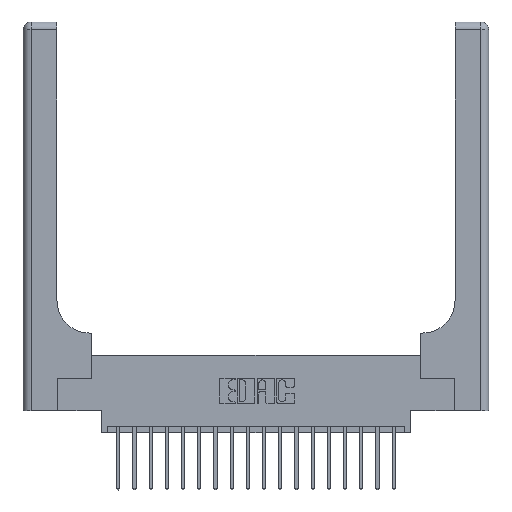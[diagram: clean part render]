
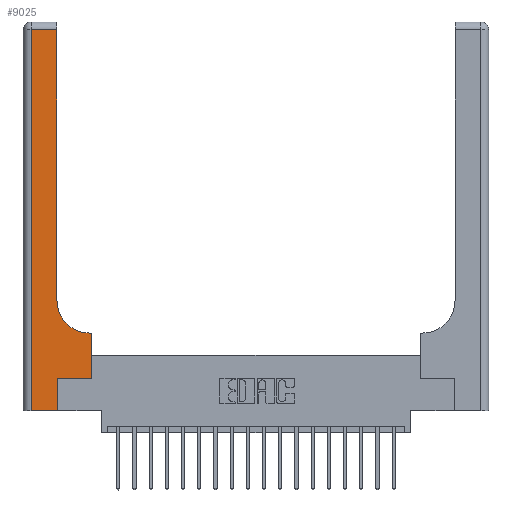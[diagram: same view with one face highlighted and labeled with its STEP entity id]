
A CAD part, top view. The second image highlights one B-rep face of the part: STEP entity #9025.
In plain terms, the highlighted planar face has unit normal (0, 0, 1).
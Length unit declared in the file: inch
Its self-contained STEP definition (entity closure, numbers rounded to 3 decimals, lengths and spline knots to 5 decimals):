
#177 = EDGE_CURVE ( 'NONE', #2294, #756, #17933, .T. ) ;
#245 = ORIENTED_EDGE ( 'NONE', *, *, #177, .T. ) ;
#266 = LINE ( 'NONE', #13153, #3987 ) ;
#305 = ORIENTED_EDGE ( 'NONE', *, *, #6806, .T. ) ;
#371 = DIRECTION ( 'NONE',  ( -1., 0., 0. ) ) ;
#756 = VERTEX_POINT ( 'NONE', #12969 ) ;
#1200 = DIRECTION ( 'NONE',  ( 0., 1., 0. ) ) ;
#1264 = LINE ( 'NONE', #1899, #4488 ) ;
#1735 = ORIENTED_EDGE ( 'NONE', *, *, #10854, .T. ) ;
#1805 = EDGE_CURVE ( 'NONE', #5435, #8838, #7093, .T. ) ;
#1899 = CARTESIAN_POINT ( 'NONE',  ( 0.265, 0., 0.37 ) ) ;
#2203 = FACE_OUTER_BOUND ( 'NONE', #16864, .T. ) ;
#2268 = CARTESIAN_POINT ( 'NONE',  ( 0.26, 3., 0.37 ) ) ;
#2294 = VERTEX_POINT ( 'NONE', #4159 ) ;
#2356 = VERTEX_POINT ( 'NONE', #2706 ) ;
#2543 = VECTOR ( 'NONE', #1200, 39.37008 ) ;
#2706 = CARTESIAN_POINT ( 'NONE',  ( 0.528, 0.6, 0.37 ) ) ;
#3165 = CARTESIAN_POINT ( 'NONE',  ( 0., 0., 0.37 ) ) ;
#3231 = AXIS2_PLACEMENT_3D ( 'NONE', #14033, #4565, #15611 ) ;
#3403 = ORIENTED_EDGE ( 'NONE', *, *, #1805, .T. ) ;
#3987 = VECTOR ( 'NONE', #6947, 39.37008 ) ;
#4159 = CARTESIAN_POINT ( 'NONE',  ( 0.06, 0., 0.37 ) ) ;
#4437 = ORIENTED_EDGE ( 'NONE', *, *, #13581, .T. ) ;
#4488 = VECTOR ( 'NONE', #14534, 39.37008 ) ;
#4565 = DIRECTION ( 'NONE',  ( 0., 0., -1. ) ) ;
#4690 = CARTESIAN_POINT ( 'NONE',  ( 0.528, 0.25, 0.37 ) ) ;
#5315 = ORIENTED_EDGE ( 'NONE', *, *, #5547, .T. ) ;
#5354 = VERTEX_POINT ( 'NONE', #15827 ) ;
#5435 = VERTEX_POINT ( 'NONE', #17510 ) ;
#5547 = EDGE_CURVE ( 'NONE', #10465, #5354, #266, .T. ) ;
#6719 = CARTESIAN_POINT ( 'NONE',  ( 0., 3., 0.37 ) ) ;
#6806 = EDGE_CURVE ( 'NONE', #756, #5435, #1264, .T. ) ;
#6947 = DIRECTION ( 'NONE',  ( -1., 0., 0. ) ) ;
#7093 = LINE ( 'NONE', #8245, #14954 ) ;
#7417 = ORIENTED_EDGE ( 'NONE', *, *, #19306, .T. ) ;
#8245 = CARTESIAN_POINT ( 'NONE',  ( 0.265, 0.25, 0.37 ) ) ;
#8731 = CARTESIAN_POINT ( 'NONE',  ( 0.51, 0.6, 0.37 ) ) ;
#8739 = EDGE_CURVE ( 'NONE', #5354, #2294, #15521, .T. ) ;
#8838 = VERTEX_POINT ( 'NONE', #4690 ) ;
#9025 = ADVANCED_FACE ( 'NONE', ( #2203 ), #19211, .F. ) ;
#9890 = DIRECTION ( 'NONE',  ( 0., 0., -1. ) ) ;
#10465 = VERTEX_POINT ( 'NONE', #12042 ) ;
#10700 = CARTESIAN_POINT ( 'NONE',  ( 0.528, 0.25, 0.37 ) ) ;
#10791 = DIRECTION ( 'NONE',  ( 0., -1., 0. ) ) ;
#10808 = LINE ( 'NONE', #2268, #14003 ) ;
#10854 = EDGE_CURVE ( 'NONE', #16754, #12481, #12821, .T. ) ;
#11356 = VECTOR ( 'NONE', #10791, 39.37008 ) ;
#11518 = ORIENTED_EDGE ( 'NONE', *, *, #19669, .T. ) ;
#12042 = CARTESIAN_POINT ( 'NONE',  ( 0.26, 2.94, 0.37 ) ) ;
#12481 = VERTEX_POINT ( 'NONE', #19895 ) ;
#12821 = CIRCLE ( 'NONE', #3231, 0.25 ) ;
#12969 = CARTESIAN_POINT ( 'NONE',  ( 0.265, 0., 0.37 ) ) ;
#13153 = CARTESIAN_POINT ( 'NONE',  ( 0., 2.94, 0.37 ) ) ;
#13317 = VECTOR ( 'NONE', #17280, 39.37008 ) ;
#13581 = EDGE_CURVE ( 'NONE', #8838, #2356, #14654, .T. ) ;
#14003 = VECTOR ( 'NONE', #16402, 39.37008 ) ;
#14033 = CARTESIAN_POINT ( 'NONE',  ( 0.51, 0.85, 0.37 ) ) ;
#14534 = DIRECTION ( 'NONE',  ( 0., 1., 0. ) ) ;
#14654 = LINE ( 'NONE', #10700, #2543 ) ;
#14703 = ORIENTED_EDGE ( 'NONE', *, *, #8739, .T. ) ;
#14954 = VECTOR ( 'NONE', #19207, 39.37008 ) ;
#15521 = LINE ( 'NONE', #18551, #11356 ) ;
#15611 = DIRECTION ( 'NONE',  ( 1., 0., 0. ) ) ;
#15827 = CARTESIAN_POINT ( 'NONE',  ( 0.06, 2.94, 0.37 ) ) ;
#16168 = AXIS2_PLACEMENT_3D ( 'NONE', #6719, #9890, #371 ) ;
#16402 = DIRECTION ( 'NONE',  ( 0., 1., 0. ) ) ;
#16754 = VERTEX_POINT ( 'NONE', #8731 ) ;
#16864 = EDGE_LOOP ( 'NONE', ( #7417, #5315, #14703, #245, #305, #3403, #4437, #11518, #1735 ) ) ;
#17274 = DIRECTION ( 'NONE',  ( -1., 0., 0. ) ) ;
#17280 = DIRECTION ( 'NONE',  ( 1., 0., 0. ) ) ;
#17510 = CARTESIAN_POINT ( 'NONE',  ( 0.265, 0.25, 0.37 ) ) ;
#17933 = LINE ( 'NONE', #3165, #13317 ) ;
#18551 = CARTESIAN_POINT ( 'NONE',  ( 0.06, 3., 0.37 ) ) ;
#18794 = CARTESIAN_POINT ( 'NONE',  ( 0.26, 0.6, 0.37 ) ) ;
#19207 = DIRECTION ( 'NONE',  ( 1., 0., 0. ) ) ;
#19211 = PLANE ( 'NONE',  #16168 ) ;
#19306 = EDGE_CURVE ( 'NONE', #12481, #10465, #10808, .T. ) ;
#19534 = VECTOR ( 'NONE', #17274, 39.37008 ) ;
#19669 = EDGE_CURVE ( 'NONE', #2356, #16754, #20012, .T. ) ;
#19895 = CARTESIAN_POINT ( 'NONE',  ( 0.26, 0.85, 0.37 ) ) ;
#20012 = LINE ( 'NONE', #18794, #19534 ) ;
